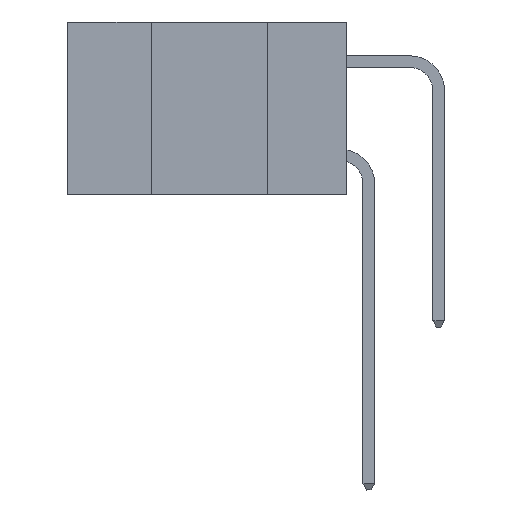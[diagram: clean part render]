
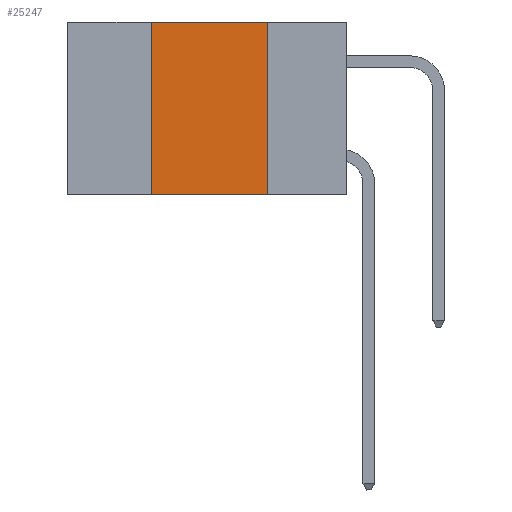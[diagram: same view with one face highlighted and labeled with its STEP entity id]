
A CAD part, left-side view. The second image highlights one B-rep face of the part: STEP entity #25247.
In plain terms, the highlighted planar face has unit normal (-1, 0, 0).
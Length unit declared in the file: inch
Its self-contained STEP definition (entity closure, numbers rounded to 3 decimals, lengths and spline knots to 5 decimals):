
#1035 = CARTESIAN_POINT ( 'NONE',  ( 0., 0.6, -0.37 ) ) ;
#1160 = EDGE_CURVE ( 'NONE', #16700, #36771, #35124, .T. ) ;
#3510 = ORIENTED_EDGE ( 'NONE', *, *, #34239, .T. ) ;
#3730 = VECTOR ( 'NONE', #27538, 39.37008 ) ;
#5099 = VERTEX_POINT ( 'NONE', #29370 ) ;
#5132 = VECTOR ( 'NONE', #9147, 39.37008 ) ;
#5196 = ORIENTED_EDGE ( 'NONE', *, *, #31705, .F. ) ;
#6727 = ORIENTED_EDGE ( 'NONE', *, *, #1160, .F. ) ;
#7503 = ORIENTED_EDGE ( 'NONE', *, *, #40606, .F. ) ;
#8760 = CARTESIAN_POINT ( 'NONE',  ( 0., 0.6, 0. ) ) ;
#9147 = DIRECTION ( 'NONE',  ( 0., -1., 0. ) ) ;
#12022 = LINE ( 'NONE', #26741, #34618 ) ;
#13923 = CARTESIAN_POINT ( 'NONE',  ( 0., 0.42, -0.37 ) ) ;
#14706 = DIRECTION ( 'NONE',  ( 0., 0., -1. ) ) ;
#16700 = VERTEX_POINT ( 'NONE', #13923 ) ;
#23781 = LINE ( 'NONE', #30830, #5132 ) ;
#25247 = ADVANCED_FACE ( 'NONE', ( #40377 ), #36647, .F. ) ;
#26099 = EDGE_LOOP ( 'NONE', ( #7503, #5196, #6727, #3510 ) ) ;
#26741 = CARTESIAN_POINT ( 'NONE',  ( 0., 0.17, 0. ) ) ;
#27227 = DIRECTION ( 'NONE',  ( 0., 0., -1. ) ) ;
#27538 = DIRECTION ( 'NONE',  ( 0., 0., 1. ) ) ;
#27553 = VECTOR ( 'NONE', #38031, 39.37008 ) ;
#28835 = VERTEX_POINT ( 'NONE', #39797 ) ;
#29370 = CARTESIAN_POINT ( 'NONE',  ( 0., 0.17, 0. ) ) ;
#30188 = CARTESIAN_POINT ( 'NONE',  ( 0., 0.42, 0. ) ) ;
#30830 = CARTESIAN_POINT ( 'NONE',  ( 0., 0.6, 0. ) ) ;
#31705 = EDGE_CURVE ( 'NONE', #36771, #5099, #23781, .T. ) ;
#32568 = AXIS2_PLACEMENT_3D ( 'NONE', #8760, #33337, #27227 ) ;
#33337 = DIRECTION ( 'NONE',  ( 1., 0., 0. ) ) ;
#34239 = EDGE_CURVE ( 'NONE', #16700, #28835, #34967, .T. ) ;
#34618 = VECTOR ( 'NONE', #14706, 39.37008 ) ;
#34967 = LINE ( 'NONE', #1035, #27553 ) ;
#35124 = LINE ( 'NONE', #30188, #3730 ) ;
#36647 = PLANE ( 'NONE',  #32568 ) ;
#36771 = VERTEX_POINT ( 'NONE', #39089 ) ;
#38031 = DIRECTION ( 'NONE',  ( 0., -1., 0. ) ) ;
#39089 = CARTESIAN_POINT ( 'NONE',  ( 0., 0.42, 0. ) ) ;
#39797 = CARTESIAN_POINT ( 'NONE',  ( 0., 0.17, -0.37 ) ) ;
#40377 = FACE_OUTER_BOUND ( 'NONE', #26099, .T. ) ;
#40606 = EDGE_CURVE ( 'NONE', #5099, #28835, #12022, .T. ) ;
